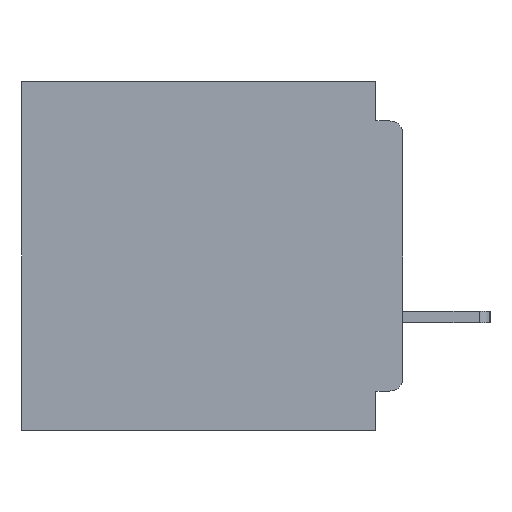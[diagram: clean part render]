
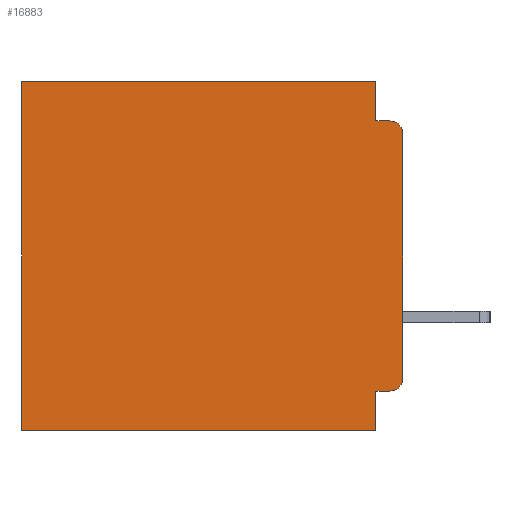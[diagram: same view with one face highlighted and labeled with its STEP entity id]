
A CAD part, left-side view. The second image highlights one B-rep face of the part: STEP entity #16883.
In plain terms, the highlighted planar face has unit normal (-1, 0, 0).
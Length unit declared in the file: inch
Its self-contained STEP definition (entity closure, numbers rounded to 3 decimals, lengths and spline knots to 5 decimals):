
#521 = VERTEX_POINT ( 'NONE', #4761 ) ;
#760 = VECTOR ( 'NONE', #30921, 39.37008 ) ;
#1297 = CARTESIAN_POINT ( 'NONE',  ( 0.3, 0.031, -0.4 ) ) ;
#1331 = FACE_OUTER_BOUND ( 'NONE', #52076, .T. ) ;
#1681 = VECTOR ( 'NONE', #46307, 39.37008 ) ;
#1821 = CARTESIAN_POINT ( 'NONE',  ( 0.3, 0., -0.4 ) ) ;
#4562 = CARTESIAN_POINT ( 'NONE',  ( 0.3, 0.015, -0.06 ) ) ;
#4761 = CARTESIAN_POINT ( 'NONE',  ( 0.3, 0.031, 0. ) ) ;
#5302 = LINE ( 'NONE', #52930, #16225 ) ;
#5527 = VERTEX_POINT ( 'NONE', #45994 ) ;
#5747 = CARTESIAN_POINT ( 'NONE',  ( 0.3, 0.031, 0. ) ) ;
#5966 = DIRECTION ( 'NONE',  ( 1., 0., 0. ) ) ;
#6012 = ORIENTED_EDGE ( 'NONE', *, *, #31878, .F. ) ;
#6517 = EDGE_CURVE ( 'NONE', #23688, #52309, #5302, .T. ) ;
#6571 = VERTEX_POINT ( 'NONE', #45177 ) ;
#6899 = DIRECTION ( 'NONE',  ( 0., 1., 0. ) ) ;
#7151 = DIRECTION ( 'NONE',  ( 0., 0., -1. ) ) ;
#8690 = DIRECTION ( 'NONE',  ( 0., 0., -1. ) ) ;
#9876 = DIRECTION ( 'NONE',  ( 0., 0., -1. ) ) ;
#10152 = DIRECTION ( 'NONE',  ( -1., 0., 0. ) ) ;
#11341 = LINE ( 'NONE', #17527, #1681 ) ;
#11494 = CARTESIAN_POINT ( 'NONE',  ( 0.3, 0.031, -0.4 ) ) ;
#11720 = LINE ( 'NONE', #26787, #760 ) ;
#15614 = DIRECTION ( 'NONE',  ( 0., 0., -1. ) ) ;
#15950 = LINE ( 'NONE', #5747, #24305 ) ;
#16225 = VECTOR ( 'NONE', #32403, 39.37008 ) ;
#16883 = ADVANCED_FACE ( 'NONE', ( #1331 ), #26469, .F. ) ;
#17424 = CARTESIAN_POINT ( 'NONE',  ( 0.3, 0.031, -0.045 ) ) ;
#17527 = CARTESIAN_POINT ( 'NONE',  ( 0.3, 0., -0.355 ) ) ;
#19133 = CARTESIAN_POINT ( 'NONE',  ( 0.3, 0.437, -0.4 ) ) ;
#19241 = ORIENTED_EDGE ( 'NONE', *, *, #51969, .F. ) ;
#19359 = CARTESIAN_POINT ( 'NONE',  ( 0.3, 0., -0.4 ) ) ;
#19750 = ORIENTED_EDGE ( 'NONE', *, *, #25833, .F. ) ;
#20610 = EDGE_CURVE ( 'NONE', #6571, #35393, #40904, .T. ) ;
#21281 = ORIENTED_EDGE ( 'NONE', *, *, #24534, .F. ) ;
#21360 = VECTOR ( 'NONE', #6899, 39.37008 ) ;
#21513 = LINE ( 'NONE', #11494, #42126 ) ;
#23111 = ORIENTED_EDGE ( 'NONE', *, *, #35271, .F. ) ;
#23248 = CARTESIAN_POINT ( 'NONE',  ( 0.3, 0., 0. ) ) ;
#23688 = VERTEX_POINT ( 'NONE', #1297 ) ;
#24305 = VECTOR ( 'NONE', #9876, 39.37008 ) ;
#24534 = EDGE_CURVE ( 'NONE', #6571, #53012, #42838, .T. ) ;
#25583 = ORIENTED_EDGE ( 'NONE', *, *, #20610, .T. ) ;
#25593 = CARTESIAN_POINT ( 'NONE',  ( 0.3, 0.437, 0. ) ) ;
#25833 = EDGE_CURVE ( 'NONE', #5527, #23688, #21513, .T. ) ;
#26469 = PLANE ( 'NONE',  #41852 ) ;
#26787 = CARTESIAN_POINT ( 'NONE',  ( 0.3, 0., -0.045 ) ) ;
#27039 = VERTEX_POINT ( 'NONE', #27482 ) ;
#27482 = CARTESIAN_POINT ( 'NONE',  ( 0.3, 0.015, -0.355 ) ) ;
#29567 = EDGE_CURVE ( 'NONE', #521, #51199, #32294, .T. ) ;
#30726 = ORIENTED_EDGE ( 'NONE', *, *, #46711, .T. ) ;
#30921 = DIRECTION ( 'NONE',  ( 0., -1., 0. ) ) ;
#31289 = ORIENTED_EDGE ( 'NONE', *, *, #29567, .T. ) ;
#31875 = VECTOR ( 'NONE', #7151, 39.37008 ) ;
#31878 = EDGE_CURVE ( 'NONE', #521, #33948, #15950, .T. ) ;
#32294 = LINE ( 'NONE', #23248, #21360 ) ;
#32403 = DIRECTION ( 'NONE',  ( 0., 1., 0. ) ) ;
#33322 = DIRECTION ( 'NONE',  ( -1., 0., 0. ) ) ;
#33339 = LINE ( 'NONE', #19133, #43046 ) ;
#33845 = CARTESIAN_POINT ( 'NONE',  ( 0.3, 0., -0.34 ) ) ;
#33948 = VERTEX_POINT ( 'NONE', #17424 ) ;
#34721 = DIRECTION ( 'NONE',  ( 0., 0., -1. ) ) ;
#34770 = CARTESIAN_POINT ( 'NONE',  ( 0.3, 0.015, -0.34 ) ) ;
#35271 = EDGE_CURVE ( 'NONE', #27039, #5527, #11341, .T. ) ;
#35393 = VERTEX_POINT ( 'NONE', #46854 ) ;
#38936 = DIRECTION ( 'NONE',  ( 0., 0., -1. ) ) ;
#40057 = ORIENTED_EDGE ( 'NONE', *, *, #6517, .F. ) ;
#40266 = AXIS2_PLACEMENT_3D ( 'NONE', #34770, #10152, #38936 ) ;
#40904 = CIRCLE ( 'NONE', #42331, 0.015 ) ;
#41852 = AXIS2_PLACEMENT_3D ( 'NONE', #1821, #5966, #34721 ) ;
#42126 = VECTOR ( 'NONE', #15614, 39.37008 ) ;
#42331 = AXIS2_PLACEMENT_3D ( 'NONE', #4562, #33322, #8690 ) ;
#42838 = LINE ( 'NONE', #19359, #31875 ) ;
#43046 = VECTOR ( 'NONE', #43964, 39.37008 ) ;
#43964 = DIRECTION ( 'NONE',  ( 0., 0., -1. ) ) ;
#45177 = CARTESIAN_POINT ( 'NONE',  ( 0.3, 0., -0.06 ) ) ;
#45994 = CARTESIAN_POINT ( 'NONE',  ( 0.3, 0.031, -0.355 ) ) ;
#46307 = DIRECTION ( 'NONE',  ( 0., 1., 0. ) ) ;
#46711 = EDGE_CURVE ( 'NONE', #27039, #53012, #49611, .T. ) ;
#46854 = CARTESIAN_POINT ( 'NONE',  ( 0.3, 0.015, -0.045 ) ) ;
#48680 = EDGE_CURVE ( 'NONE', #51199, #52309, #33339, .T. ) ;
#49611 = CIRCLE ( 'NONE', #40266, 0.015 ) ;
#49758 = CARTESIAN_POINT ( 'NONE',  ( 0.3, 0.437, -0.4 ) ) ;
#50779 = ORIENTED_EDGE ( 'NONE', *, *, #48680, .T. ) ;
#51199 = VERTEX_POINT ( 'NONE', #25593 ) ;
#51969 = EDGE_CURVE ( 'NONE', #33948, #35393, #11720, .T. ) ;
#52076 = EDGE_LOOP ( 'NONE', ( #21281, #25583, #19241, #6012, #31289, #50779, #40057, #19750, #23111, #30726 ) ) ;
#52309 = VERTEX_POINT ( 'NONE', #49758 ) ;
#52930 = CARTESIAN_POINT ( 'NONE',  ( 0.3, 0., -0.4 ) ) ;
#53012 = VERTEX_POINT ( 'NONE', #33845 ) ;
